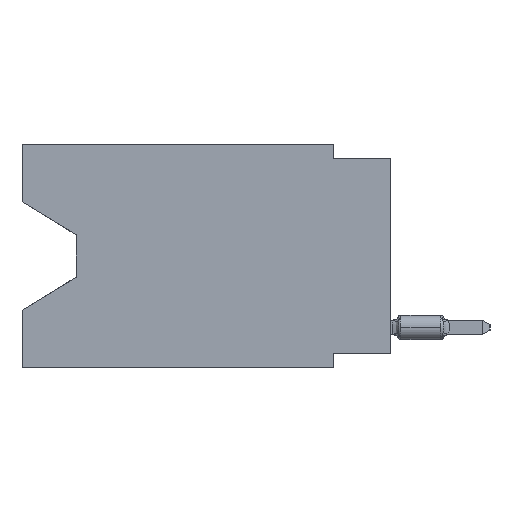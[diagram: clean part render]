
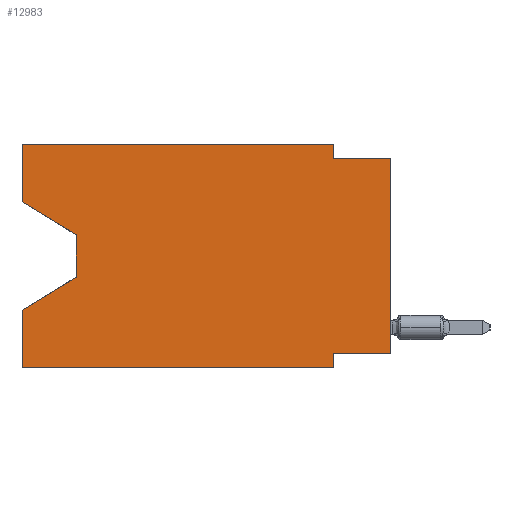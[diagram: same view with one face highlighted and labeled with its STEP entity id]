
A CAD part, left-side view. The second image highlights one B-rep face of the part: STEP entity #12983.
In plain terms, the highlighted planar face has unit normal (-1, 0, 0).
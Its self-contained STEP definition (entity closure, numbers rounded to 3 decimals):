
#410 = VECTOR ( 'NONE', #12375, 1000. ) ;
#1138 = VECTOR ( 'NONE', #21447, 1000. ) ;
#1383 = EDGE_CURVE ( 'NONE', #16659, #19604, #21037, .T. ) ;
#1814 = CARTESIAN_POINT ( 'NONE',  ( 0., 0., -0.635 ) ) ;
#1933 = EDGE_CURVE ( 'NONE', #19604, #14921, #3379, .T. ) ;
#2263 = LINE ( 'NONE', #19737, #2954 ) ;
#2401 = CARTESIAN_POINT ( 'NONE',  ( 0., 16.383, 0. ) ) ;
#2417 = DIRECTION ( 'NONE',  ( 0., 0., -1. ) ) ;
#2440 = EDGE_CURVE ( 'NONE', #21093, #3061, #11190, .T. ) ;
#2811 = ORIENTED_EDGE ( 'NONE', *, *, #17681, .F. ) ;
#2881 = VECTOR ( 'NONE', #13471, 1000. ) ;
#2893 = VERTEX_POINT ( 'NONE', #14910 ) ;
#2954 = VECTOR ( 'NONE', #3971, 1000. ) ;
#3005 = CARTESIAN_POINT ( 'NONE',  ( 0., 16.383, 0. ) ) ;
#3061 = VERTEX_POINT ( 'NONE', #20796 ) ;
#3115 = DIRECTION ( 'NONE',  ( 0., 0., 1. ) ) ;
#3212 = ORIENTED_EDGE ( 'NONE', *, *, #11977, .F. ) ;
#3379 = LINE ( 'NONE', #6564, #2881 ) ;
#3876 = ORIENTED_EDGE ( 'NONE', *, *, #2440, .T. ) ;
#3971 = DIRECTION ( 'NONE',  ( 0., 0., -1. ) ) ;
#4749 = ORIENTED_EDGE ( 'NONE', *, *, #4868, .F. ) ;
#4760 = VECTOR ( 'NONE', #16786, 1000. ) ;
#4868 = EDGE_CURVE ( 'NONE', #8640, #11354, #10802, .T. ) ;
#4901 = CARTESIAN_POINT ( 'NONE',  ( 0., 2.54, 0. ) ) ;
#5362 = ORIENTED_EDGE ( 'NONE', *, *, #1933, .F. ) ;
#5432 = VECTOR ( 'NONE', #3115, 1000. ) ;
#5495 = CARTESIAN_POINT ( 'NONE',  ( 0., 2.54, -9.271 ) ) ;
#6057 = DIRECTION ( 'NONE',  ( 0., 0., 1. ) ) ;
#6071 = CARTESIAN_POINT ( 'NONE',  ( 0., 16.383, -2.546 ) ) ;
#6564 = CARTESIAN_POINT ( 'NONE',  ( 0., 2.54, 0. ) ) ;
#6755 = CARTESIAN_POINT ( 'NONE',  ( 0., 0., -9.271 ) ) ;
#7265 = CARTESIAN_POINT ( 'NONE',  ( 0., 0., 0. ) ) ;
#8245 = LINE ( 'NONE', #3005, #5432 ) ;
#8640 = VERTEX_POINT ( 'NONE', #16367 ) ;
#8911 = EDGE_LOOP ( 'NONE', ( #3876, #12702, #13583, #4749, #16836, #2811, #3212, #20109, #17183, #5362, #18324, #20011 ) ) ;
#8953 = LINE ( 'NONE', #7265, #18147 ) ;
#8995 = CARTESIAN_POINT ( 'NONE',  ( 0., 16.383, -9.906 ) ) ;
#9688 = FACE_OUTER_BOUND ( 'NONE', #8911, .T. ) ;
#9749 = AXIS2_PLACEMENT_3D ( 'NONE', #16701, #18296, #2417 ) ;
#9809 = VECTOR ( 'NONE', #19942, 1000. ) ;
#10439 = LINE ( 'NONE', #1814, #10597 ) ;
#10597 = VECTOR ( 'NONE', #14059, 1000. ) ;
#10802 = LINE ( 'NONE', #2401, #16063 ) ;
#11190 = LINE ( 'NONE', #21390, #11943 ) ;
#11354 = VERTEX_POINT ( 'NONE', #19813 ) ;
#11418 = VERTEX_POINT ( 'NONE', #11423 ) ;
#11423 = CARTESIAN_POINT ( 'NONE',  ( 0., 13.97, -5.893 ) ) ;
#11943 = VECTOR ( 'NONE', #16422, 1000. ) ;
#11977 = EDGE_CURVE ( 'NONE', #22410, #16698, #19611, .T. ) ;
#12076 = EDGE_CURVE ( 'NONE', #3061, #11418, #15066, .T. ) ;
#12375 = DIRECTION ( 'NONE',  ( 0., 1., 0. ) ) ;
#12560 = CARTESIAN_POINT ( 'NONE',  ( 0., 16.383, 0. ) ) ;
#12702 = ORIENTED_EDGE ( 'NONE', *, *, #12076, .T. ) ;
#12983 = ADVANCED_FACE ( 'NONE', ( #9688 ), #21808, .F. ) ;
#13286 = EDGE_CURVE ( 'NONE', #21093, #16659, #8245, .T. ) ;
#13471 = DIRECTION ( 'NONE',  ( 0., 0., -1. ) ) ;
#13583 = ORIENTED_EDGE ( 'NONE', *, *, #15109, .T. ) ;
#14059 = DIRECTION ( 'NONE',  ( 0., -1., 0. ) ) ;
#14357 = DIRECTION ( 'NONE',  ( 0., -1., 0. ) ) ;
#14631 = CARTESIAN_POINT ( 'NONE',  ( 0., 0., -9.271 ) ) ;
#14910 = CARTESIAN_POINT ( 'NONE',  ( 0., 2.54, -9.906 ) ) ;
#14921 = VERTEX_POINT ( 'NONE', #21861 ) ;
#15066 = LINE ( 'NONE', #18568, #9809 ) ;
#15109 = EDGE_CURVE ( 'NONE', #11418, #11354, #21984, .T. ) ;
#15118 = VERTEX_POINT ( 'NONE', #17111 ) ;
#15228 = EDGE_CURVE ( 'NONE', #22410, #15118, #8953, .T. ) ;
#16063 = VECTOR ( 'NONE', #6057, 1000. ) ;
#16367 = CARTESIAN_POINT ( 'NONE',  ( 0., 16.383, -9.906 ) ) ;
#16422 = DIRECTION ( 'NONE',  ( 0., -0.855, -0.519 ) ) ;
#16659 = VERTEX_POINT ( 'NONE', #21232 ) ;
#16698 = VERTEX_POINT ( 'NONE', #5495 ) ;
#16701 = CARTESIAN_POINT ( 'NONE',  ( 0., 16.383, 0. ) ) ;
#16786 = DIRECTION ( 'NONE',  ( 0., 0.855, -0.519 ) ) ;
#16836 = ORIENTED_EDGE ( 'NONE', *, *, #17294, .T. ) ;
#17111 = CARTESIAN_POINT ( 'NONE',  ( 0., 0., -0.635 ) ) ;
#17183 = ORIENTED_EDGE ( 'NONE', *, *, #21872, .F. ) ;
#17294 = EDGE_CURVE ( 'NONE', #8640, #2893, #19418, .T. ) ;
#17681 = EDGE_CURVE ( 'NONE', #16698, #2893, #2263, .T. ) ;
#18147 = VECTOR ( 'NONE', #21069, 1000. ) ;
#18296 = DIRECTION ( 'NONE',  ( 1., 0., 0. ) ) ;
#18324 = ORIENTED_EDGE ( 'NONE', *, *, #1383, .F. ) ;
#18568 = CARTESIAN_POINT ( 'NONE',  ( 0., 13.97, -4.013 ) ) ;
#19418 = LINE ( 'NONE', #8995, #1138 ) ;
#19604 = VERTEX_POINT ( 'NONE', #4901 ) ;
#19611 = LINE ( 'NONE', #14631, #410 ) ;
#19737 = CARTESIAN_POINT ( 'NONE',  ( 0., 2.54, -9.906 ) ) ;
#19813 = CARTESIAN_POINT ( 'NONE',  ( 0., 16.383, -7.36 ) ) ;
#19878 = VECTOR ( 'NONE', #14357, 1000. ) ;
#19942 = DIRECTION ( 'NONE',  ( 0., 0., -1. ) ) ;
#20011 = ORIENTED_EDGE ( 'NONE', *, *, #13286, .F. ) ;
#20109 = ORIENTED_EDGE ( 'NONE', *, *, #15228, .T. ) ;
#20517 = CARTESIAN_POINT ( 'NONE',  ( 0., 13.97, -5.893 ) ) ;
#20796 = CARTESIAN_POINT ( 'NONE',  ( 0., 13.97, -4.013 ) ) ;
#21037 = LINE ( 'NONE', #12560, #19878 ) ;
#21069 = DIRECTION ( 'NONE',  ( 0., 0., 1. ) ) ;
#21093 = VERTEX_POINT ( 'NONE', #6071 ) ;
#21232 = CARTESIAN_POINT ( 'NONE',  ( 0., 16.383, 0. ) ) ;
#21390 = CARTESIAN_POINT ( 'NONE',  ( 0., 16.383, -2.546 ) ) ;
#21447 = DIRECTION ( 'NONE',  ( 0., -1., 0. ) ) ;
#21808 = PLANE ( 'NONE',  #9749 ) ;
#21861 = CARTESIAN_POINT ( 'NONE',  ( 0., 2.54, -0.635 ) ) ;
#21872 = EDGE_CURVE ( 'NONE', #14921, #15118, #10439, .T. ) ;
#21984 = LINE ( 'NONE', #20517, #4760 ) ;
#22410 = VERTEX_POINT ( 'NONE', #6755 ) ;
